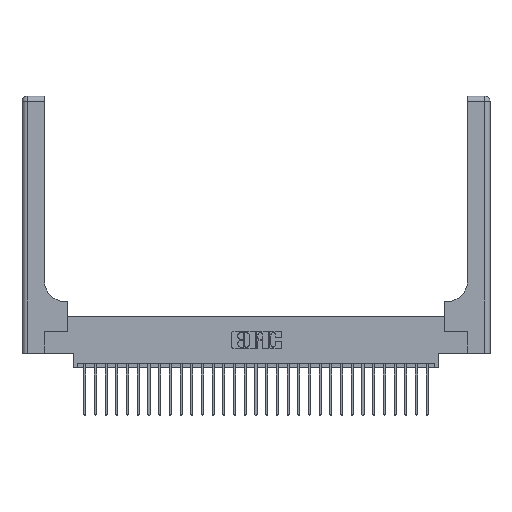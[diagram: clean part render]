
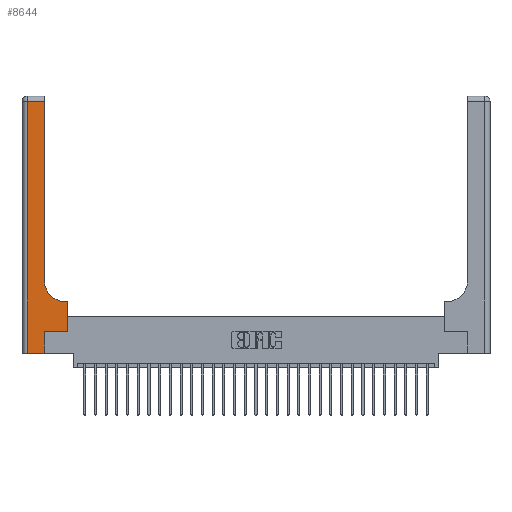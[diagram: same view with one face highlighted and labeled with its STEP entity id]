
A CAD part, top view. The second image highlights one B-rep face of the part: STEP entity #8644.
In plain terms, the highlighted planar face has unit normal (0, 0, 1).
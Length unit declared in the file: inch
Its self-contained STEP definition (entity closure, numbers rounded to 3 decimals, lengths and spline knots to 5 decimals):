
#107 = ORIENTED_EDGE ( 'NONE', *, *, #3020, .T. ) ;
#755 = CIRCLE ( 'NONE', #16888, 0.25 ) ;
#930 = CARTESIAN_POINT ( 'NONE',  ( 0.265, 0., 0.37 ) ) ;
#1190 = DIRECTION ( 'NONE',  ( 0., 0., -1. ) ) ;
#2524 = VERTEX_POINT ( 'NONE', #10683 ) ;
#2660 = EDGE_CURVE ( 'NONE', #16351, #18332, #21320, .T. ) ;
#2806 = DIRECTION ( 'NONE',  ( 1., 0., 0. ) ) ;
#3020 = EDGE_CURVE ( 'NONE', #24878, #22673, #755, .T. ) ;
#4237 = ORIENTED_EDGE ( 'NONE', *, *, #13968, .T. ) ;
#4288 = CARTESIAN_POINT ( 'NONE',  ( 0., 0., 0.37 ) ) ;
#5133 = EDGE_CURVE ( 'NONE', #10212, #13895, #7895, .T. ) ;
#5977 = VECTOR ( 'NONE', #28409, 39.37008 ) ;
#6317 = LINE ( 'NONE', #4288, #5977 ) ;
#6349 = CARTESIAN_POINT ( 'NONE',  ( 0.26, 3., 0.37 ) ) ;
#6379 = VECTOR ( 'NONE', #26262, 39.37008 ) ;
#6454 = LINE ( 'NONE', #26085, #7556 ) ;
#7017 = EDGE_CURVE ( 'NONE', #2524, #16351, #6454, .T. ) ;
#7279 = DIRECTION ( 'NONE',  ( 0., 1., 0. ) ) ;
#7556 = VECTOR ( 'NONE', #2806, 39.37008 ) ;
#7770 = DIRECTION ( 'NONE',  ( -1., 0., 0. ) ) ;
#7816 = CARTESIAN_POINT ( 'NONE',  ( 0.51, 0.85, 0.37 ) ) ;
#7895 = LINE ( 'NONE', #9925, #22816 ) ;
#8047 = LINE ( 'NONE', #21037, #15079 ) ;
#8049 = LINE ( 'NONE', #21319, #23985 ) ;
#8566 = VERTEX_POINT ( 'NONE', #10600 ) ;
#8592 = CARTESIAN_POINT ( 'NONE',  ( 0.528, 0.25, 0.37 ) ) ;
#8644 = ADVANCED_FACE ( 'NONE', ( #19405 ), #12639, .F. ) ;
#8662 = CARTESIAN_POINT ( 'NONE',  ( 0.06, 0., 0.37 ) ) ;
#9796 = ORIENTED_EDGE ( 'NONE', *, *, #16830, .T. ) ;
#9925 = CARTESIAN_POINT ( 'NONE',  ( 0., 2.94, 0.37 ) ) ;
#10212 = VERTEX_POINT ( 'NONE', #19245 ) ;
#10406 = VECTOR ( 'NONE', #15380, 39.37008 ) ;
#10600 = CARTESIAN_POINT ( 'NONE',  ( 0.265, 0., 0.37 ) ) ;
#10660 = LINE ( 'NONE', #6349, #6379 ) ;
#10683 = CARTESIAN_POINT ( 'NONE',  ( 0.265, 0.25, 0.37 ) ) ;
#12639 = PLANE ( 'NONE',  #12667 ) ;
#12667 = AXIS2_PLACEMENT_3D ( 'NONE', #21148, #18856, #21424 ) ;
#13895 = VERTEX_POINT ( 'NONE', #18743 ) ;
#13968 = EDGE_CURVE ( 'NONE', #18332, #24878, #8047, .T. ) ;
#14073 = LINE ( 'NONE', #930, #23865 ) ;
#14326 = DIRECTION ( 'NONE',  ( 1., 0., 0. ) ) ;
#14838 = EDGE_CURVE ( 'NONE', #8566, #2524, #14073, .T. ) ;
#15075 = ORIENTED_EDGE ( 'NONE', *, *, #7017, .T. ) ;
#15079 = VECTOR ( 'NONE', #7770, 39.37008 ) ;
#15104 = EDGE_CURVE ( 'NONE', #22673, #10212, #10660, .T. ) ;
#15380 = DIRECTION ( 'NONE',  ( 0., 1., 0. ) ) ;
#15515 = CARTESIAN_POINT ( 'NONE',  ( 0.51, 0.6, 0.37 ) ) ;
#16351 = VERTEX_POINT ( 'NONE', #21352 ) ;
#16830 = EDGE_CURVE ( 'NONE', #22618, #8566, #6317, .T. ) ;
#16888 = AXIS2_PLACEMENT_3D ( 'NONE', #7816, #1190, #14326 ) ;
#17965 = EDGE_CURVE ( 'NONE', #13895, #22618, #8049, .T. ) ;
#18332 = VERTEX_POINT ( 'NONE', #27384 ) ;
#18743 = CARTESIAN_POINT ( 'NONE',  ( 0.06, 2.94, 0.37 ) ) ;
#18856 = DIRECTION ( 'NONE',  ( 0., 0., -1. ) ) ;
#19245 = CARTESIAN_POINT ( 'NONE',  ( 0.26, 2.94, 0.37 ) ) ;
#19405 = FACE_OUTER_BOUND ( 'NONE', #22334, .T. ) ;
#19941 = ORIENTED_EDGE ( 'NONE', *, *, #17965, .T. ) ;
#21037 = CARTESIAN_POINT ( 'NONE',  ( 0.26, 0.6, 0.37 ) ) ;
#21148 = CARTESIAN_POINT ( 'NONE',  ( 0., 3., 0.37 ) ) ;
#21177 = DIRECTION ( 'NONE',  ( 0., -1., 0. ) ) ;
#21319 = CARTESIAN_POINT ( 'NONE',  ( 0.06, 3., 0.37 ) ) ;
#21320 = LINE ( 'NONE', #8592, #10406 ) ;
#21352 = CARTESIAN_POINT ( 'NONE',  ( 0.528, 0.25, 0.37 ) ) ;
#21424 = DIRECTION ( 'NONE',  ( -1., 0., 0. ) ) ;
#21839 = ORIENTED_EDGE ( 'NONE', *, *, #5133, .T. ) ;
#22334 = EDGE_LOOP ( 'NONE', ( #24005, #21839, #19941, #9796, #27245, #15075, #25747, #4237, #107 ) ) ;
#22618 = VERTEX_POINT ( 'NONE', #8662 ) ;
#22673 = VERTEX_POINT ( 'NONE', #23946 ) ;
#22816 = VECTOR ( 'NONE', #22911, 39.37008 ) ;
#22911 = DIRECTION ( 'NONE',  ( -1., 0., 0. ) ) ;
#23865 = VECTOR ( 'NONE', #7279, 39.37008 ) ;
#23946 = CARTESIAN_POINT ( 'NONE',  ( 0.26, 0.85, 0.37 ) ) ;
#23985 = VECTOR ( 'NONE', #21177, 39.37008 ) ;
#24005 = ORIENTED_EDGE ( 'NONE', *, *, #15104, .T. ) ;
#24878 = VERTEX_POINT ( 'NONE', #15515 ) ;
#25747 = ORIENTED_EDGE ( 'NONE', *, *, #2660, .T. ) ;
#26085 = CARTESIAN_POINT ( 'NONE',  ( 0.265, 0.25, 0.37 ) ) ;
#26262 = DIRECTION ( 'NONE',  ( 0., 1., 0. ) ) ;
#27245 = ORIENTED_EDGE ( 'NONE', *, *, #14838, .T. ) ;
#27384 = CARTESIAN_POINT ( 'NONE',  ( 0.528, 0.6, 0.37 ) ) ;
#28409 = DIRECTION ( 'NONE',  ( 1., 0., 0. ) ) ;
